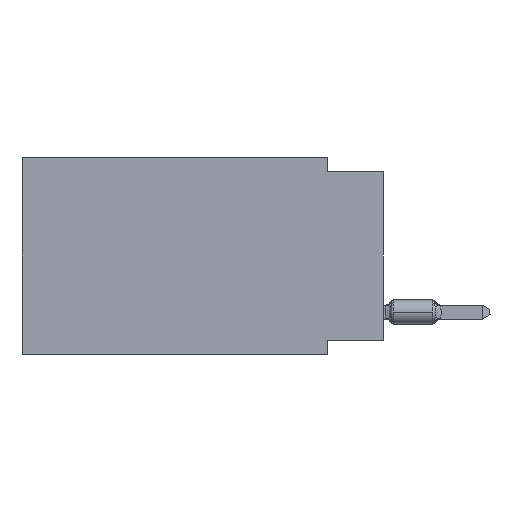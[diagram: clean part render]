
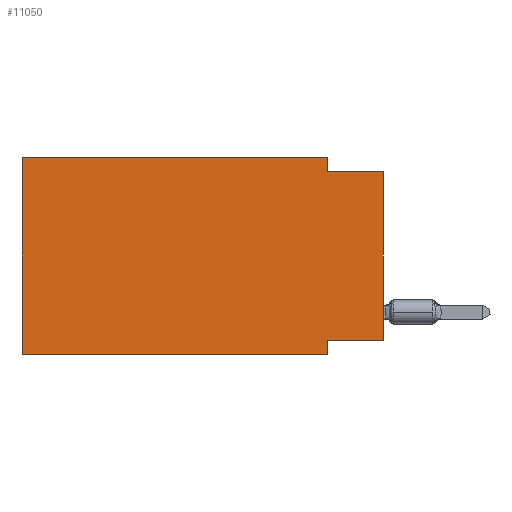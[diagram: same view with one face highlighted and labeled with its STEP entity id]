
A CAD part, left-side view. The second image highlights one B-rep face of the part: STEP entity #11050.
In plain terms, the highlighted planar face has unit normal (-1, 0, 0).
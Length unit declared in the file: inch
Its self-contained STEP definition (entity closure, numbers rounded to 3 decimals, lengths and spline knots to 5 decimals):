
#251 = CARTESIAN_POINT ( 'NONE',  ( 0., 0., -0.325 ) ) ;
#1238 = DIRECTION ( 'NONE',  ( 0., 1., 0. ) ) ;
#1450 = CARTESIAN_POINT ( 'NONE',  ( 0., 0.645, -0.35 ) ) ;
#2162 = CARTESIAN_POINT ( 'NONE',  ( 0., 0.1, 0. ) ) ;
#2165 = VECTOR ( 'NONE', #23897, 39.37008 ) ;
#2297 = VERTEX_POINT ( 'NONE', #4256 ) ;
#4256 = CARTESIAN_POINT ( 'NONE',  ( 0., 0.645, 0. ) ) ;
#4413 = DIRECTION ( 'NONE',  ( 1., 0., 0. ) ) ;
#4500 = VERTEX_POINT ( 'NONE', #22651 ) ;
#5296 = LINE ( 'NONE', #12405, #6750 ) ;
#5625 = LINE ( 'NONE', #8212, #12447 ) ;
#5834 = VECTOR ( 'NONE', #16822, 39.37008 ) ;
#6750 = VECTOR ( 'NONE', #9981, 39.37008 ) ;
#7042 = CARTESIAN_POINT ( 'NONE',  ( 0., 0.645, 0. ) ) ;
#7339 = CARTESIAN_POINT ( 'NONE',  ( 0., 0.645, 0. ) ) ;
#8094 = AXIS2_PLACEMENT_3D ( 'NONE', #7339, #4413, #19326 ) ;
#8175 = DIRECTION ( 'NONE',  ( 0., 0., 1. ) ) ;
#8212 = CARTESIAN_POINT ( 'NONE',  ( 0., 0., 0. ) ) ;
#8287 = ORIENTED_EDGE ( 'NONE', *, *, #23227, .T. ) ;
#8397 = LINE ( 'NONE', #23591, #23065 ) ;
#8630 = CARTESIAN_POINT ( 'NONE',  ( 0., 0.1, -0.35 ) ) ;
#8891 = VERTEX_POINT ( 'NONE', #18906 ) ;
#9981 = DIRECTION ( 'NONE',  ( 0., -1., 0. ) ) ;
#10237 = VERTEX_POINT ( 'NONE', #251 ) ;
#10870 = VECTOR ( 'NONE', #8175, 39.37008 ) ;
#10914 = VERTEX_POINT ( 'NONE', #8630 ) ;
#11050 = ADVANCED_FACE ( 'NONE', ( #31626 ), #29517, .F. ) ;
#11841 = VECTOR ( 'NONE', #21556, 39.37008 ) ;
#12296 = LINE ( 'NONE', #29026, #11841 ) ;
#12405 = CARTESIAN_POINT ( 'NONE',  ( 0., 0.645, -0.35 ) ) ;
#12447 = VECTOR ( 'NONE', #18093, 39.37008 ) ;
#13043 = EDGE_CURVE ( 'NONE', #10237, #30006, #8397, .T. ) ;
#13109 = CARTESIAN_POINT ( 'NONE',  ( 0., 0.1, -0.325 ) ) ;
#15622 = VERTEX_POINT ( 'NONE', #1450 ) ;
#16264 = ORIENTED_EDGE ( 'NONE', *, *, #25012, .T. ) ;
#16609 = LINE ( 'NONE', #7042, #16640 ) ;
#16640 = VECTOR ( 'NONE', #28741, 39.37008 ) ;
#16822 = DIRECTION ( 'NONE',  ( 0., 0., -1. ) ) ;
#17539 = EDGE_CURVE ( 'NONE', #8891, #4500, #12296, .T. ) ;
#17755 = ORIENTED_EDGE ( 'NONE', *, *, #26553, .F. ) ;
#18093 = DIRECTION ( 'NONE',  ( 0., 0., 1. ) ) ;
#18906 = CARTESIAN_POINT ( 'NONE',  ( 0., 0.1, -0.025 ) ) ;
#18992 = VERTEX_POINT ( 'NONE', #28019 ) ;
#19192 = LINE ( 'NONE', #2162, #2165 ) ;
#19241 = ORIENTED_EDGE ( 'NONE', *, *, #13043, .F. ) ;
#19260 = LINE ( 'NONE', #24105, #5834 ) ;
#19326 = DIRECTION ( 'NONE',  ( 0., 0., -1. ) ) ;
#19847 = EDGE_LOOP ( 'NONE', ( #8287, #29995, #17755, #26413, #31927, #16264, #27095, #19241 ) ) ;
#21556 = DIRECTION ( 'NONE',  ( 0., -1., 0. ) ) ;
#22333 = CARTESIAN_POINT ( 'NONE',  ( 0., 0.645, 0. ) ) ;
#22651 = CARTESIAN_POINT ( 'NONE',  ( 0., 0., -0.025 ) ) ;
#23065 = VECTOR ( 'NONE', #1238, 39.37008 ) ;
#23227 = EDGE_CURVE ( 'NONE', #10237, #4500, #5625, .T. ) ;
#23431 = EDGE_CURVE ( 'NONE', #15622, #2297, #30349, .T. ) ;
#23591 = CARTESIAN_POINT ( 'NONE',  ( 0., 0., -0.325 ) ) ;
#23897 = DIRECTION ( 'NONE',  ( 0., 0., -1. ) ) ;
#24105 = CARTESIAN_POINT ( 'NONE',  ( 0., 0.1, -0.35 ) ) ;
#25012 = EDGE_CURVE ( 'NONE', #15622, #10914, #5296, .T. ) ;
#26413 = ORIENTED_EDGE ( 'NONE', *, *, #31190, .F. ) ;
#26553 = EDGE_CURVE ( 'NONE', #18992, #8891, #19192, .T. ) ;
#27095 = ORIENTED_EDGE ( 'NONE', *, *, #27381, .F. ) ;
#27381 = EDGE_CURVE ( 'NONE', #30006, #10914, #19260, .T. ) ;
#28019 = CARTESIAN_POINT ( 'NONE',  ( 0., 0.1, 0. ) ) ;
#28741 = DIRECTION ( 'NONE',  ( 0., -1., 0. ) ) ;
#29026 = CARTESIAN_POINT ( 'NONE',  ( 0., 0., -0.025 ) ) ;
#29517 = PLANE ( 'NONE',  #8094 ) ;
#29995 = ORIENTED_EDGE ( 'NONE', *, *, #17539, .F. ) ;
#30006 = VERTEX_POINT ( 'NONE', #13109 ) ;
#30349 = LINE ( 'NONE', #22333, #10870 ) ;
#31190 = EDGE_CURVE ( 'NONE', #2297, #18992, #16609, .T. ) ;
#31626 = FACE_OUTER_BOUND ( 'NONE', #19847, .T. ) ;
#31927 = ORIENTED_EDGE ( 'NONE', *, *, #23431, .F. ) ;
